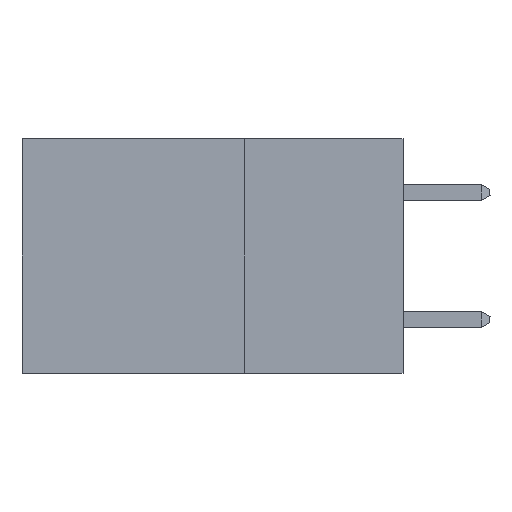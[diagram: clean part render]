
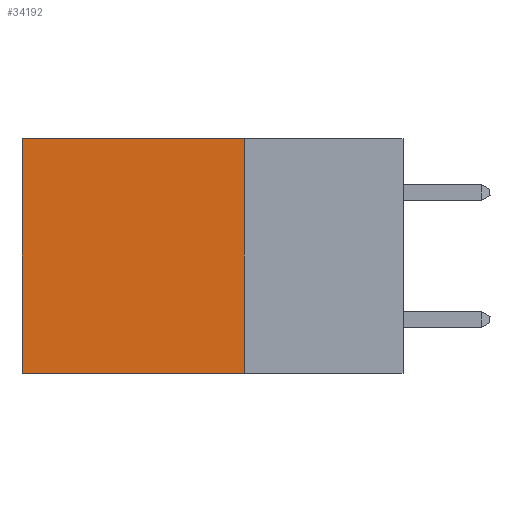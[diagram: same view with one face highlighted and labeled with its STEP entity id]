
A CAD part, left-side view. The second image highlights one B-rep face of the part: STEP entity #34192.
In plain terms, the highlighted planar face has unit normal (-1, 0, 0).
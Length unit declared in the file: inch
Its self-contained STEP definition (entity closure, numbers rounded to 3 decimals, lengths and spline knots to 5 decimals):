
#125 = EDGE_LOOP ( 'NONE', ( #43141, #36782, #11731, #24150 ) ) ;
#163 = LINE ( 'NONE', #15939, #14960 ) ;
#2678 = CARTESIAN_POINT ( 'NONE',  ( 0.2875, 0.25, 0. ) ) ;
#3420 = DIRECTION ( 'NONE',  ( 1., 0., 0. ) ) ;
#5460 = VERTEX_POINT ( 'NONE', #10361 ) ;
#6429 = EDGE_CURVE ( 'NONE', #22381, #5460, #163, .T. ) ;
#6920 = EDGE_CURVE ( 'NONE', #22381, #11385, #24720, .T. ) ;
#8085 = CARTESIAN_POINT ( 'NONE',  ( 0.2875, 0.25, 0. ) ) ;
#10361 = CARTESIAN_POINT ( 'NONE',  ( 0.2875, 0.6, 0. ) ) ;
#11385 = VERTEX_POINT ( 'NONE', #18709 ) ;
#11731 = ORIENTED_EDGE ( 'NONE', *, *, #6920, .F. ) ;
#13860 = PLANE ( 'NONE',  #27937 ) ;
#14741 = LINE ( 'NONE', #32074, #19605 ) ;
#14960 = VECTOR ( 'NONE', #26006, 39.37008 ) ;
#15475 = VECTOR ( 'NONE', #40720, 39.37008 ) ;
#15939 = CARTESIAN_POINT ( 'NONE',  ( 0.2875, 0.25, 0. ) ) ;
#17028 = FACE_OUTER_BOUND ( 'NONE', #125, .T. ) ;
#18709 = CARTESIAN_POINT ( 'NONE',  ( 0.2875, 0.25, -0.37 ) ) ;
#18925 = DIRECTION ( 'NONE',  ( 0., 1., 0. ) ) ;
#19126 = EDGE_CURVE ( 'NONE', #5460, #41201, #41928, .T. ) ;
#19605 = VECTOR ( 'NONE', #18925, 39.37008 ) ;
#20695 = DIRECTION ( 'NONE',  ( 0., 0., -1. ) ) ;
#22381 = VERTEX_POINT ( 'NONE', #8085 ) ;
#24150 = ORIENTED_EDGE ( 'NONE', *, *, #6429, .T. ) ;
#24720 = LINE ( 'NONE', #2678, #15475 ) ;
#26006 = DIRECTION ( 'NONE',  ( 0., 1., 0. ) ) ;
#27859 = CARTESIAN_POINT ( 'NONE',  ( 0.2875, 0.25, 0. ) ) ;
#27937 = AXIS2_PLACEMENT_3D ( 'NONE', #27859, #3420, #20695 ) ;
#29578 = CARTESIAN_POINT ( 'NONE',  ( 0.2875, 0.6, -0.37 ) ) ;
#30302 = DIRECTION ( 'NONE',  ( 0., 0., -1. ) ) ;
#32074 = CARTESIAN_POINT ( 'NONE',  ( 0.2875, 0.25, -0.37 ) ) ;
#34192 = ADVANCED_FACE ( 'NONE', ( #17028 ), #13860, .F. ) ;
#36239 = EDGE_CURVE ( 'NONE', #11385, #41201, #14741, .T. ) ;
#36782 = ORIENTED_EDGE ( 'NONE', *, *, #36239, .F. ) ;
#37473 = CARTESIAN_POINT ( 'NONE',  ( 0.2875, 0.6, 0. ) ) ;
#39762 = VECTOR ( 'NONE', #30302, 39.37008 ) ;
#40720 = DIRECTION ( 'NONE',  ( 0., 0., -1. ) ) ;
#41201 = VERTEX_POINT ( 'NONE', #29578 ) ;
#41928 = LINE ( 'NONE', #37473, #39762 ) ;
#43141 = ORIENTED_EDGE ( 'NONE', *, *, #19126, .T. ) ;
